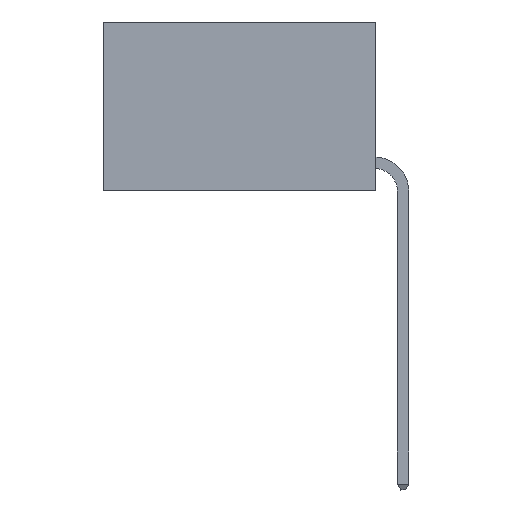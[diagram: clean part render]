
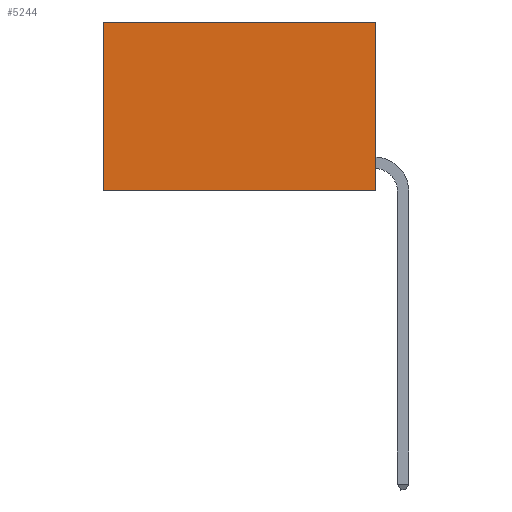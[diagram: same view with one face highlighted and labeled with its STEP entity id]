
A CAD part, left-side view. The second image highlights one B-rep face of the part: STEP entity #5244.
In plain terms, the highlighted planar face has unit normal (-1, 0, 0).
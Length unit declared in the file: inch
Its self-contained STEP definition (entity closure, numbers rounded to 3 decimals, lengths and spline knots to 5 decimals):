
#54 = CARTESIAN_POINT ( 'NONE',  ( 0.2625, 0.6, -0.37 ) ) ;
#193 = CARTESIAN_POINT ( 'NONE',  ( 0.2625, 0., 0. ) ) ;
#289 = ORIENTED_EDGE ( 'NONE', *, *, #9246, .T. ) ;
#626 = ORIENTED_EDGE ( 'NONE', *, *, #4421, .F. ) ;
#756 = ORIENTED_EDGE ( 'NONE', *, *, #2846, .T. ) ;
#792 = LINE ( 'NONE', #3565, #6398 ) ;
#977 = AXIS2_PLACEMENT_3D ( 'NONE', #4908, #5477, #8445 ) ;
#1120 = CARTESIAN_POINT ( 'NONE',  ( 0.2625, 0., 0. ) ) ;
#1808 = DIRECTION ( 'NONE',  ( 0., 1., 0. ) ) ;
#2410 = VERTEX_POINT ( 'NONE', #3573 ) ;
#2581 = PLANE ( 'NONE',  #977 ) ;
#2846 = EDGE_CURVE ( 'NONE', #2410, #6788, #792, .T. ) ;
#3340 = VERTEX_POINT ( 'NONE', #3508 ) ;
#3508 = CARTESIAN_POINT ( 'NONE',  ( 0.2625, 0., 0. ) ) ;
#3565 = CARTESIAN_POINT ( 'NONE',  ( 0.2625, 0.6, 0. ) ) ;
#3573 = CARTESIAN_POINT ( 'NONE',  ( 0.2625, 0.6, 0. ) ) ;
#3610 = DIRECTION ( 'NONE',  ( 0., 0., -1. ) ) ;
#3844 = LINE ( 'NONE', #193, #6298 ) ;
#3995 = DIRECTION ( 'NONE',  ( 0., 1., 0. ) ) ;
#4172 = CARTESIAN_POINT ( 'NONE',  ( 0.2625, 0., -0.37 ) ) ;
#4244 = EDGE_CURVE ( 'NONE', #3340, #6182, #3844, .T. ) ;
#4421 = EDGE_CURVE ( 'NONE', #6182, #6788, #6296, .T. ) ;
#4686 = LINE ( 'NONE', #1120, #6290 ) ;
#4790 = ORIENTED_EDGE ( 'NONE', *, *, #4244, .F. ) ;
#4908 = CARTESIAN_POINT ( 'NONE',  ( 0.2625, 0., 0. ) ) ;
#5244 = ADVANCED_FACE ( 'NONE', ( #8527 ), #2581, .F. ) ;
#5477 = DIRECTION ( 'NONE',  ( 1., 0., 0. ) ) ;
#5813 = VECTOR ( 'NONE', #1808, 39.37008 ) ;
#6182 = VERTEX_POINT ( 'NONE', #4172 ) ;
#6290 = VECTOR ( 'NONE', #3995, 39.37008 ) ;
#6296 = LINE ( 'NONE', #8432, #5813 ) ;
#6298 = VECTOR ( 'NONE', #8102, 39.37008 ) ;
#6398 = VECTOR ( 'NONE', #3610, 39.37008 ) ;
#6788 = VERTEX_POINT ( 'NONE', #54 ) ;
#7697 = EDGE_LOOP ( 'NONE', ( #756, #626, #4790, #289 ) ) ;
#8102 = DIRECTION ( 'NONE',  ( 0., 0., -1. ) ) ;
#8432 = CARTESIAN_POINT ( 'NONE',  ( 0.2625, 0., -0.37 ) ) ;
#8445 = DIRECTION ( 'NONE',  ( 0., 0., -1. ) ) ;
#8527 = FACE_OUTER_BOUND ( 'NONE', #7697, .T. ) ;
#9246 = EDGE_CURVE ( 'NONE', #3340, #2410, #4686, .T. ) ;
